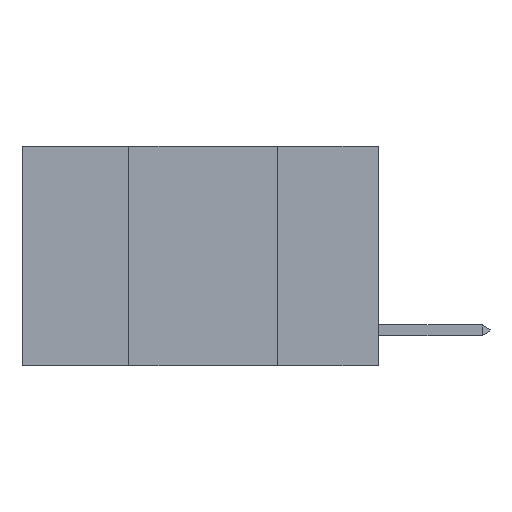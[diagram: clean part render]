
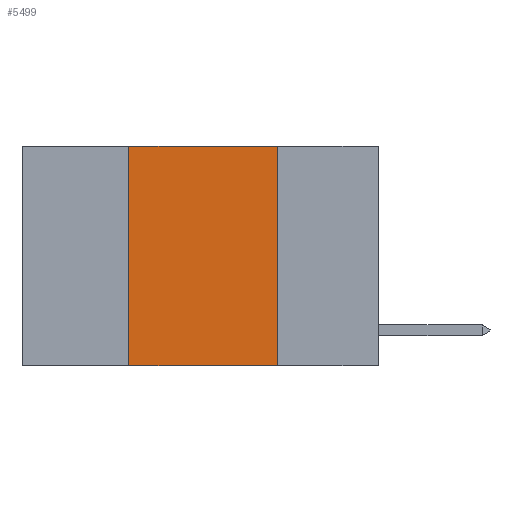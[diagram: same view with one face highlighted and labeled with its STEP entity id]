
A CAD part, left-side view. The second image highlights one B-rep face of the part: STEP entity #5499.
In plain terms, the highlighted planar face has unit normal (-1, 0, 0).
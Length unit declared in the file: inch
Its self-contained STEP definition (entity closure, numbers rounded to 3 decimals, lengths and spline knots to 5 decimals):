
#378 = CARTESIAN_POINT ( 'NONE',  ( 0., 0.6, -0.37 ) ) ;
#506 = ORIENTED_EDGE ( 'NONE', *, *, #5832, .F. ) ;
#1038 = LINE ( 'NONE', #5400, #1606 ) ;
#1606 = VECTOR ( 'NONE', #4433, 39.37008 ) ;
#1805 = DIRECTION ( 'NONE',  ( 0., 0., -1. ) ) ;
#1959 = DIRECTION ( 'NONE',  ( 0., 0., -1. ) ) ;
#3183 = VERTEX_POINT ( 'NONE', #13980 ) ;
#3250 = LINE ( 'NONE', #8660, #8014 ) ;
#3431 = CARTESIAN_POINT ( 'NONE',  ( 0., 0.42, 0. ) ) ;
#3935 = VECTOR ( 'NONE', #1959, 39.37008 ) ;
#4232 = CARTESIAN_POINT ( 'NONE',  ( 0., 0.17, -0.37 ) ) ;
#4311 = VERTEX_POINT ( 'NONE', #3431 ) ;
#4433 = DIRECTION ( 'NONE',  ( 0., 0., 1. ) ) ;
#5135 = CARTESIAN_POINT ( 'NONE',  ( 0., 0.42, -0.37 ) ) ;
#5400 = CARTESIAN_POINT ( 'NONE',  ( 0., 0.42, 0. ) ) ;
#5495 = VERTEX_POINT ( 'NONE', #5135 ) ;
#5499 = ADVANCED_FACE ( 'NONE', ( #8556 ), #13059, .F. ) ;
#5832 = EDGE_CURVE ( 'NONE', #3183, #14320, #11954, .T. ) ;
#5843 = VECTOR ( 'NONE', #12504, 39.37008 ) ;
#6852 = EDGE_CURVE ( 'NONE', #5495, #14320, #6875, .T. ) ;
#6875 = LINE ( 'NONE', #378, #5843 ) ;
#7441 = DIRECTION ( 'NONE',  ( 1., 0., 0. ) ) ;
#8014 = VECTOR ( 'NONE', #8871, 39.37008 ) ;
#8033 = EDGE_CURVE ( 'NONE', #5495, #4311, #1038, .T. ) ;
#8556 = FACE_OUTER_BOUND ( 'NONE', #10749, .T. ) ;
#8660 = CARTESIAN_POINT ( 'NONE',  ( 0., 0.6, 0. ) ) ;
#8871 = DIRECTION ( 'NONE',  ( 0., -1., 0. ) ) ;
#9119 = AXIS2_PLACEMENT_3D ( 'NONE', #10761, #7441, #1805 ) ;
#10341 = EDGE_CURVE ( 'NONE', #4311, #3183, #3250, .T. ) ;
#10749 = EDGE_LOOP ( 'NONE', ( #506, #12835, #10969, #12371 ) ) ;
#10761 = CARTESIAN_POINT ( 'NONE',  ( 0., 0.6, 0. ) ) ;
#10969 = ORIENTED_EDGE ( 'NONE', *, *, #8033, .F. ) ;
#11954 = LINE ( 'NONE', #14085, #3935 ) ;
#12371 = ORIENTED_EDGE ( 'NONE', *, *, #6852, .T. ) ;
#12504 = DIRECTION ( 'NONE',  ( 0., -1., 0. ) ) ;
#12835 = ORIENTED_EDGE ( 'NONE', *, *, #10341, .F. ) ;
#13059 = PLANE ( 'NONE',  #9119 ) ;
#13980 = CARTESIAN_POINT ( 'NONE',  ( 0., 0.17, 0. ) ) ;
#14085 = CARTESIAN_POINT ( 'NONE',  ( 0., 0.17, 0. ) ) ;
#14320 = VERTEX_POINT ( 'NONE', #4232 ) ;
